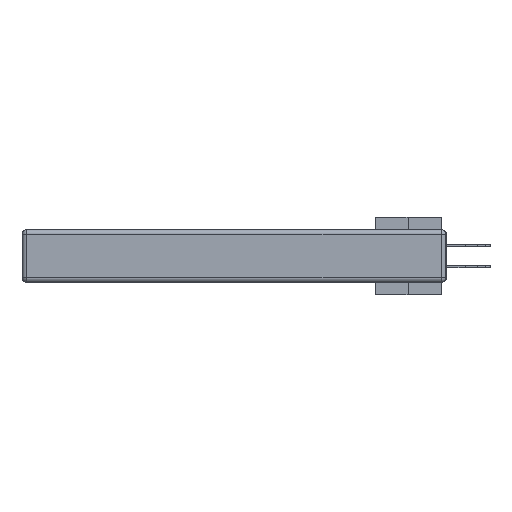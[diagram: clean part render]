
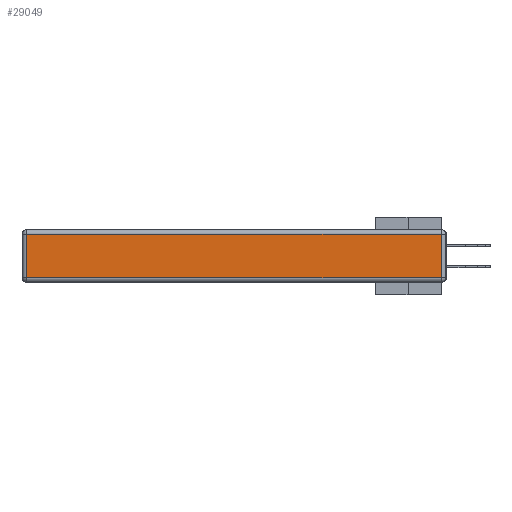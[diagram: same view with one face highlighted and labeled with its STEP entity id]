
A CAD part, left-side view. The second image highlights one B-rep face of the part: STEP entity #29049.
In plain terms, the highlighted planar face has unit normal (-1, 0, 0).
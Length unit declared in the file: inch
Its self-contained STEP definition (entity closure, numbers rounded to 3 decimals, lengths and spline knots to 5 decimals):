
#3842 = PLANE ( 'NONE',  #13386 ) ;
#5557 = DIRECTION ( 'NONE',  ( 0., 1., 0. ) ) ;
#6944 = FACE_OUTER_BOUND ( 'NONE', #7111, .T. ) ;
#7111 = EDGE_LOOP ( 'NONE', ( #21164, #30731, #7925, #32728 ) ) ;
#7925 = ORIENTED_EDGE ( 'NONE', *, *, #13784, .T. ) ;
#9544 = VECTOR ( 'NONE', #5557, 39.37008 ) ;
#11737 = VECTOR ( 'NONE', #12923, 39.37008 ) ;
#12180 = VERTEX_POINT ( 'NONE', #20807 ) ;
#12923 = DIRECTION ( 'NONE',  ( 0., 0., 1. ) ) ;
#13386 = AXIS2_PLACEMENT_3D ( 'NONE', #34945, #17992, #23461 ) ;
#13784 = EDGE_CURVE ( 'NONE', #18405, #12180, #21487, .T. ) ;
#13888 = VERTEX_POINT ( 'NONE', #34006 ) ;
#13917 = LINE ( 'NONE', #14329, #25414 ) ;
#14329 = CARTESIAN_POINT ( 'NONE',  ( 0., 0., -0.313 ) ) ;
#15321 = CARTESIAN_POINT ( 'NONE',  ( 0., 2.72, -0.343 ) ) ;
#17401 = DIRECTION ( 'NONE',  ( 0., -1., 0. ) ) ;
#17604 = VECTOR ( 'NONE', #35130, 39.37008 ) ;
#17992 = DIRECTION ( 'NONE',  ( -1., 0., 0. ) ) ;
#18317 = EDGE_CURVE ( 'NONE', #12180, #13888, #26898, .T. ) ;
#18405 = VERTEX_POINT ( 'NONE', #27431 ) ;
#20138 = EDGE_CURVE ( 'NONE', #25582, #18405, #28563, .T. ) ;
#20807 = CARTESIAN_POINT ( 'NONE',  ( 0., 2.72, -0.03 ) ) ;
#21164 = ORIENTED_EDGE ( 'NONE', *, *, #30726, .T. ) ;
#21487 = LINE ( 'NONE', #23494, #9544 ) ;
#22567 = CARTESIAN_POINT ( 'NONE',  ( 0., 0.03, -0.313 ) ) ;
#23461 = DIRECTION ( 'NONE',  ( 0., 0., 1. ) ) ;
#23494 = CARTESIAN_POINT ( 'NONE',  ( 0., 2.75, -0.03 ) ) ;
#25414 = VECTOR ( 'NONE', #17401, 39.37008 ) ;
#25582 = VERTEX_POINT ( 'NONE', #22567 ) ;
#26898 = LINE ( 'NONE', #15321, #17604 ) ;
#27431 = CARTESIAN_POINT ( 'NONE',  ( 0., 0.03, -0.03 ) ) ;
#28563 = LINE ( 'NONE', #32085, #11737 ) ;
#29049 = ADVANCED_FACE ( 'NONE', ( #6944 ), #3842, .T. ) ;
#30726 = EDGE_CURVE ( 'NONE', #13888, #25582, #13917, .T. ) ;
#30731 = ORIENTED_EDGE ( 'NONE', *, *, #20138, .T. ) ;
#32085 = CARTESIAN_POINT ( 'NONE',  ( 0., 0.03, -0.343 ) ) ;
#32728 = ORIENTED_EDGE ( 'NONE', *, *, #18317, .T. ) ;
#34006 = CARTESIAN_POINT ( 'NONE',  ( 0., 2.72, -0.313 ) ) ;
#34945 = CARTESIAN_POINT ( 'NONE',  ( 0., 0., -0.343 ) ) ;
#35130 = DIRECTION ( 'NONE',  ( 0., 0., -1. ) ) ;
